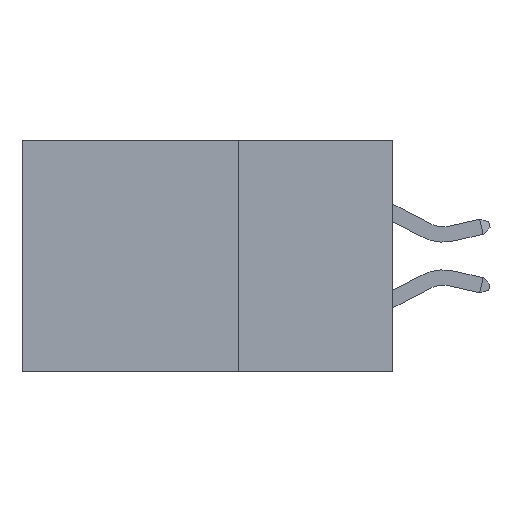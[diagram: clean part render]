
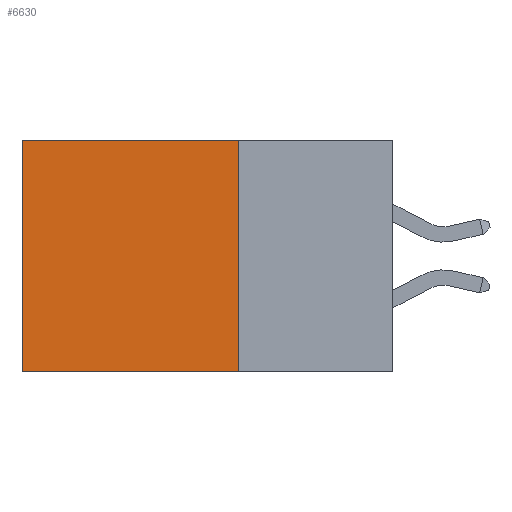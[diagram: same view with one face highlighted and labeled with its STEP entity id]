
A CAD part, left-side view. The second image highlights one B-rep face of the part: STEP entity #6630.
In plain terms, the highlighted planar face has unit normal (-1, 0, 0).
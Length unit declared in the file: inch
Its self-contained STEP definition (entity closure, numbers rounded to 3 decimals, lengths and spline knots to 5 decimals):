
#323 = DIRECTION ( 'NONE',  ( 0., 1., 0. ) ) ;
#428 = DIRECTION ( 'NONE',  ( 0., 0., -1. ) ) ;
#535 = ORIENTED_EDGE ( 'NONE', *, *, #7885, .F. ) ;
#579 = LINE ( 'NONE', #1777, #7578 ) ;
#630 = CARTESIAN_POINT ( 'NONE',  ( 0.2875, 0.6, -0.375 ) ) ;
#823 = ORIENTED_EDGE ( 'NONE', *, *, #4339, .T. ) ;
#933 = DIRECTION ( 'NONE',  ( 0., 0., -1. ) ) ;
#964 = DIRECTION ( 'NONE',  ( 1., 0., 0. ) ) ;
#1044 = AXIS2_PLACEMENT_3D ( 'NONE', #6231, #964, #933 ) ;
#1478 = PLANE ( 'NONE',  #1044 ) ;
#1671 = EDGE_LOOP ( 'NONE', ( #823, #535, #4993, #2420 ) ) ;
#1777 = CARTESIAN_POINT ( 'NONE',  ( 0.2875, 0.6, -0.375 ) ) ;
#2420 = ORIENTED_EDGE ( 'NONE', *, *, #3352, .T. ) ;
#3352 = EDGE_CURVE ( 'NONE', #7157, #4003, #7504, .T. ) ;
#3778 = VECTOR ( 'NONE', #428, 39.37008 ) ;
#4003 = VERTEX_POINT ( 'NONE', #5098 ) ;
#4118 = DIRECTION ( 'NONE',  ( 0., 1., 0. ) ) ;
#4339 = EDGE_CURVE ( 'NONE', #4003, #6492, #579, .T. ) ;
#4444 = CARTESIAN_POINT ( 'NONE',  ( 0.2875, 0.25, -0.375 ) ) ;
#4969 = CARTESIAN_POINT ( 'NONE',  ( 0.2875, 0.25, 0. ) ) ;
#4993 = ORIENTED_EDGE ( 'NONE', *, *, #8719, .F. ) ;
#5098 = CARTESIAN_POINT ( 'NONE',  ( 0.2875, 0.6, 0. ) ) ;
#5716 = CARTESIAN_POINT ( 'NONE',  ( 0.2875, 0.25, -0.375 ) ) ;
#5923 = DIRECTION ( 'NONE',  ( 0., 0., -1. ) ) ;
#6105 = LINE ( 'NONE', #5716, #7598 ) ;
#6231 = CARTESIAN_POINT ( 'NONE',  ( 0.2875, 0.25, -0.375 ) ) ;
#6492 = VERTEX_POINT ( 'NONE', #630 ) ;
#6630 = ADVANCED_FACE ( 'NONE', ( #8277 ), #1478, .F. ) ;
#6945 = VECTOR ( 'NONE', #4118, 39.37008 ) ;
#7157 = VERTEX_POINT ( 'NONE', #4969 ) ;
#7298 = VERTEX_POINT ( 'NONE', #4444 ) ;
#7475 = CARTESIAN_POINT ( 'NONE',  ( 0.2875, 0.25, 0. ) ) ;
#7504 = LINE ( 'NONE', #7475, #6945 ) ;
#7578 = VECTOR ( 'NONE', #5923, 39.37008 ) ;
#7598 = VECTOR ( 'NONE', #323, 39.37008 ) ;
#7885 = EDGE_CURVE ( 'NONE', #7298, #6492, #6105, .T. ) ;
#8277 = FACE_OUTER_BOUND ( 'NONE', #1671, .T. ) ;
#8548 = CARTESIAN_POINT ( 'NONE',  ( 0.2875, 0.25, -0.375 ) ) ;
#8719 = EDGE_CURVE ( 'NONE', #7157, #7298, #8726, .T. ) ;
#8726 = LINE ( 'NONE', #8548, #3778 ) ;
